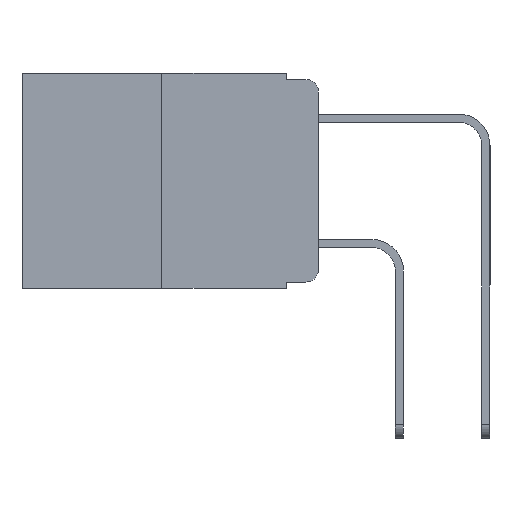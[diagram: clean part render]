
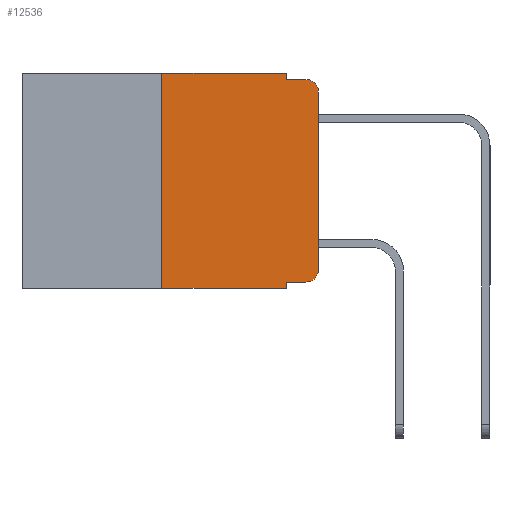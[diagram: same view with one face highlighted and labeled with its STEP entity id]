
A CAD part, left-side view. The second image highlights one B-rep face of the part: STEP entity #12536.
In plain terms, the highlighted planar face has unit normal (-1, 0, 0).
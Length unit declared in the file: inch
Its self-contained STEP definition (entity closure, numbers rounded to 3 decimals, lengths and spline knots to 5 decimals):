
#58 = VERTEX_POINT ( 'NONE', #13833 ) ;
#337 = VECTOR ( 'NONE', #15719, 39.37008 ) ;
#1044 = VECTOR ( 'NONE', #5288, 39.37008 ) ;
#1087 = VERTEX_POINT ( 'NONE', #16684 ) ;
#1104 = EDGE_CURVE ( 'NONE', #5820, #12857, #6219, .T. ) ;
#1170 = ORIENTED_EDGE ( 'NONE', *, *, #3740, .T. ) ;
#1222 = EDGE_LOOP ( 'NONE', ( #10940, #11425, #8752, #1399, #10229, #16190, #12637, #19488, #1170, #2134 ) ) ;
#1399 = ORIENTED_EDGE ( 'NONE', *, *, #16094, .F. ) ;
#1727 = DIRECTION ( 'NONE',  ( 0., 0., 1. ) ) ;
#2134 = ORIENTED_EDGE ( 'NONE', *, *, #1104, .T. ) ;
#2139 = EDGE_CURVE ( 'NONE', #1087, #9049, #17079, .T. ) ;
#2179 = DIRECTION ( 'NONE',  ( 0., 0., -1. ) ) ;
#2447 = DIRECTION ( 'NONE',  ( -1., 0., 0. ) ) ;
#2745 = VECTOR ( 'NONE', #6497, 39.37008 ) ;
#3340 = CARTESIAN_POINT ( 'NONE',  ( 0., 0.473, 0. ) ) ;
#3740 = EDGE_CURVE ( 'NONE', #1087, #5820, #16074, .T. ) ;
#4028 = DIRECTION ( 'NONE',  ( -1., 0., 0. ) ) ;
#4036 = VERTEX_POINT ( 'NONE', #17791 ) ;
#4194 = LINE ( 'NONE', #13594, #20016 ) ;
#4922 = CARTESIAN_POINT ( 'NONE',  ( 0., 0., 0. ) ) ;
#5288 = DIRECTION ( 'NONE',  ( 0., -1., 0. ) ) ;
#5340 = PLANE ( 'NONE',  #13386 ) ;
#5730 = CARTESIAN_POINT ( 'NONE',  ( 0., 0.02, -0.333 ) ) ;
#5820 = VERTEX_POINT ( 'NONE', #5730 ) ;
#6219 = CIRCLE ( 'NONE', #7564, 0.02 ) ;
#6497 = DIRECTION ( 'NONE',  ( 0., -1., 0. ) ) ;
#6784 = CARTESIAN_POINT ( 'NONE',  ( 0., 0.02, -0.01 ) ) ;
#6868 = CIRCLE ( 'NONE', #11027, 0.02 ) ;
#6903 = DIRECTION ( 'NONE',  ( 1., 0., 0. ) ) ;
#7386 = VERTEX_POINT ( 'NONE', #17355 ) ;
#7564 = AXIS2_PLACEMENT_3D ( 'NONE', #16948, #2447, #2179 ) ;
#8526 = DIRECTION ( 'NONE',  ( 0., 0., -1. ) ) ;
#8752 = ORIENTED_EDGE ( 'NONE', *, *, #14544, .F. ) ;
#8843 = VERTEX_POINT ( 'NONE', #12863 ) ;
#9049 = VERTEX_POINT ( 'NONE', #11842 ) ;
#9180 = DIRECTION ( 'NONE',  ( 0., 0., -1. ) ) ;
#10229 = ORIENTED_EDGE ( 'NONE', *, *, #10550, .F. ) ;
#10449 = CARTESIAN_POINT ( 'NONE',  ( 0., 0.051, 0. ) ) ;
#10550 = EDGE_CURVE ( 'NONE', #4036, #8843, #15119, .T. ) ;
#10774 = CARTESIAN_POINT ( 'NONE',  ( 0., 0.051, -0.01 ) ) ;
#10940 = ORIENTED_EDGE ( 'NONE', *, *, #19578, .T. ) ;
#11027 = AXIS2_PLACEMENT_3D ( 'NONE', #13323, #4028, #14836 ) ;
#11099 = CARTESIAN_POINT ( 'NONE',  ( 0., 0.25, 0. ) ) ;
#11142 = EDGE_CURVE ( 'NONE', #7386, #4036, #19796, .T. ) ;
#11425 = ORIENTED_EDGE ( 'NONE', *, *, #17066, .T. ) ;
#11842 = CARTESIAN_POINT ( 'NONE',  ( 0., 0.051, -0.343 ) ) ;
#12323 = CARTESIAN_POINT ( 'NONE',  ( 0., 0., -0.313 ) ) ;
#12536 = ADVANCED_FACE ( 'NONE', ( #18818 ), #5340, .F. ) ;
#12637 = ORIENTED_EDGE ( 'NONE', *, *, #16568, .T. ) ;
#12857 = VERTEX_POINT ( 'NONE', #12323 ) ;
#12858 = VERTEX_POINT ( 'NONE', #10774 ) ;
#12863 = CARTESIAN_POINT ( 'NONE',  ( 0., 0.051, 0. ) ) ;
#12979 = LINE ( 'NONE', #18307, #17464 ) ;
#13002 = VECTOR ( 'NONE', #14885, 39.37008 ) ;
#13027 = CARTESIAN_POINT ( 'NONE',  ( 0., 0.051, -0.01 ) ) ;
#13071 = VECTOR ( 'NONE', #8526, 39.37008 ) ;
#13290 = LINE ( 'NONE', #4922, #337 ) ;
#13323 = CARTESIAN_POINT ( 'NONE',  ( 0., 0.02, -0.03 ) ) ;
#13386 = AXIS2_PLACEMENT_3D ( 'NONE', #16114, #6903, #17620 ) ;
#13594 = CARTESIAN_POINT ( 'NONE',  ( 0., 0.473, -0.343 ) ) ;
#13833 = CARTESIAN_POINT ( 'NONE',  ( 0., 0., -0.03 ) ) ;
#14544 = EDGE_CURVE ( 'NONE', #12858, #17828, #17020, .T. ) ;
#14836 = DIRECTION ( 'NONE',  ( 0., 0., -1. ) ) ;
#14885 = DIRECTION ( 'NONE',  ( 0., -1., 0. ) ) ;
#14944 = CARTESIAN_POINT ( 'NONE',  ( 0., 0.051, -0.333 ) ) ;
#15119 = LINE ( 'NONE', #3340, #2745 ) ;
#15719 = DIRECTION ( 'NONE',  ( 0., 0., 1. ) ) ;
#16074 = LINE ( 'NONE', #14944, #13002 ) ;
#16094 = EDGE_CURVE ( 'NONE', #8843, #12858, #12979, .T. ) ;
#16114 = CARTESIAN_POINT ( 'NONE',  ( 0., 0.473, 0. ) ) ;
#16190 = ORIENTED_EDGE ( 'NONE', *, *, #11142, .F. ) ;
#16275 = VECTOR ( 'NONE', #1727, 39.37008 ) ;
#16568 = EDGE_CURVE ( 'NONE', #7386, #9049, #4194, .T. ) ;
#16684 = CARTESIAN_POINT ( 'NONE',  ( 0., 0.051, -0.333 ) ) ;
#16948 = CARTESIAN_POINT ( 'NONE',  ( 0., 0.02, -0.313 ) ) ;
#17020 = LINE ( 'NONE', #13027, #1044 ) ;
#17066 = EDGE_CURVE ( 'NONE', #58, #17828, #6868, .T. ) ;
#17079 = LINE ( 'NONE', #10449, #13071 ) ;
#17355 = CARTESIAN_POINT ( 'NONE',  ( 0., 0.25, -0.343 ) ) ;
#17464 = VECTOR ( 'NONE', #9180, 39.37008 ) ;
#17620 = DIRECTION ( 'NONE',  ( 0., 0., -1. ) ) ;
#17791 = CARTESIAN_POINT ( 'NONE',  ( 0., 0.25, 0. ) ) ;
#17828 = VERTEX_POINT ( 'NONE', #6784 ) ;
#18307 = CARTESIAN_POINT ( 'NONE',  ( 0., 0.051, 0. ) ) ;
#18818 = FACE_OUTER_BOUND ( 'NONE', #1222, .T. ) ;
#19488 = ORIENTED_EDGE ( 'NONE', *, *, #2139, .F. ) ;
#19578 = EDGE_CURVE ( 'NONE', #12857, #58, #13290, .T. ) ;
#19666 = DIRECTION ( 'NONE',  ( 0., -1., 0. ) ) ;
#19796 = LINE ( 'NONE', #11099, #16275 ) ;
#20016 = VECTOR ( 'NONE', #19666, 39.37008 ) ;
